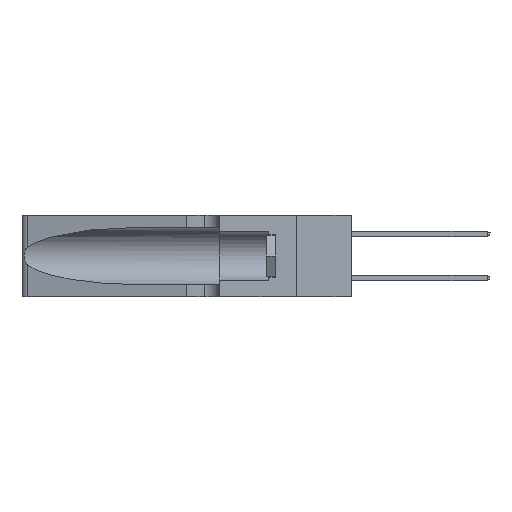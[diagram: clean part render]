
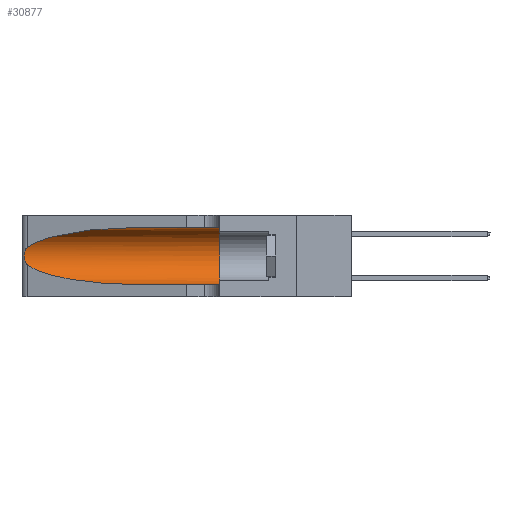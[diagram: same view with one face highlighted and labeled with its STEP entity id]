
A CAD part, left-side view. The second image highlights one B-rep face of the part: STEP entity #30877.
In plain terms, the highlighted cylindrical face has radius 3.308 mm (diameter 6.617 mm), a partial arc.
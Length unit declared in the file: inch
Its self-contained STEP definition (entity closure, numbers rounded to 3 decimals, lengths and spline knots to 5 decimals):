
#311 = CARTESIAN_POINT ( 'NONE',  ( 0.18966, 0.96281, 0.31525 ) ) ;
#879 = ORIENTED_EDGE ( 'NONE', *, *, #33293, .T. ) ;
#2165 = ORIENTED_EDGE ( 'NONE', *, *, #10543, .F. ) ;
#2223 = EDGE_CURVE ( 'NONE', #2775, #30299, #10175, .T. ) ;
#2388 = EDGE_CURVE ( 'NONE', #2775, #19255, #10539, .T. ) ;
#2775 = VERTEX_POINT ( 'NONE', #29743 ) ;
#3473 = EDGE_LOOP ( 'NONE', ( #18449, #19280, #879, #35013, #2165, #21034 ) ) ;
#5345 = CARTESIAN_POINT ( 'NONE',  ( 0.25787, 1.23484, 0.2124 ) ) ;
#5373 = DIRECTION ( 'NONE',  ( 0., -1., 0. ) ) ;
#5460 = DIRECTION ( 'NONE',  ( 0., -1., 0. ) ) ;
#7367 = CARTESIAN_POINT ( 'NONE',  ( 0.1305, 0.72297, 0.05475 ) ) ;
#8260 = CARTESIAN_POINT ( 'NONE',  ( 0.26018, 1.23835, 0.19895 ) ) ;
#8306 = CARTESIAN_POINT ( 'NONE',  ( 0.25487, 1.22718, 0.14631 ) ) ;
#9261 = CARTESIAN_POINT ( 'NONE',  ( 0.18966, 0.96281, 0.05475 ) ) ;
#9454 = FACE_OUTER_BOUND ( 'NONE', #3473, .T. ) ;
#10175 = LINE ( 'NONE', #22093, #12773 ) ;
#10539 =( BOUNDED_CURVE ( )  B_SPLINE_CURVE ( 3, ( #28117, #311, #17195, #30842 ),
 .UNSPECIFIED., .F., .F. ) 
 B_SPLINE_CURVE_WITH_KNOTS ( ( 4, 4 ),
 ( 1.5708, 2.84003 ),
 .UNSPECIFIED. ) 
 CURVE ( )  GEOMETRIC_REPRESENTATION_ITEM ( )  RATIONAL_B_SPLINE_CURVE ( ( 1., 0.87, 0.87, 1. ) ) 
 REPRESENTATION_ITEM ( '' )  );
#10543 = EDGE_CURVE ( 'NONE', #30299, #10990, #32500, .T. ) ;
#10990 = VERTEX_POINT ( 'NONE', #35467 ) ;
#11045 = CARTESIAN_POINT ( 'NONE',  ( 0.26075, 1.23896, 0.178 ) ) ;
#11640 =( BOUNDED_CURVE ( )  B_SPLINE_CURVE ( 3, ( #17498, #33737, #9261, #28424 ),
 .UNSPECIFIED., .F., .T. ) 
 B_SPLINE_CURVE_WITH_KNOTS ( ( 4, 4 ),
 ( 3.44316, 4.71239 ),
 .UNSPECIFIED. ) 
 CURVE ( )  GEOMETRIC_REPRESENTATION_ITEM ( )  RATIONAL_B_SPLINE_CURVE ( ( 1., 0.87, 0.87, 1. ) ) 
 REPRESENTATION_ITEM ( '' )  );
#11899 = AXIS2_PLACEMENT_3D ( 'NONE', #30862, #14536, #33576 ) ;
#12773 = VECTOR ( 'NONE', #5460, 39.37008 ) ;
#13812 = CARTESIAN_POINT ( 'NONE',  ( 0.25856, 1.23593, 0.16098 ) ) ;
#14536 = DIRECTION ( 'NONE',  ( 0., 1., 0. ) ) ;
#15426 = EDGE_CURVE ( 'NONE', #20231, #10990, #32007, .T. ) ;
#15476 = DIRECTION ( 'NONE',  ( 0., 0., -1. ) ) ;
#16509 = CARTESIAN_POINT ( 'NONE',  ( 0.25555, 1.22994, 0.2215 ) ) ;
#16623 = CARTESIAN_POINT ( 'NONE',  ( 0.25639, 1.23186, 0.15144 ) ) ;
#17195 = CARTESIAN_POINT ( 'NONE',  ( 0.2373, 1.15595, 0.28018 ) ) ;
#17498 = CARTESIAN_POINT ( 'NONE',  ( 0.25487, 1.22718, 0.14631 ) ) ;
#17573 = VECTOR ( 'NONE', #22804, 39.37008 ) ;
#18077 = B_SPLINE_CURVE_WITH_KNOTS ( 'NONE', 3,
 ( #19250, #16509, #21989, #5345, #24711, #8260, #27418, #11045, #30160, #13812, #32869, #16623, #35623, #19364 ),
 .UNSPECIFIED., .F., .F.,
 ( 4, 2, 2, 2, 2, 2, 4 ),
 ( 0., 0.00027, 0.00053, 0.00107, 0.0016, 0.00187, 0.00214 ),
 .UNSPECIFIED. ) ;
#18449 = ORIENTED_EDGE ( 'NONE', *, *, #2388, .T. ) ;
#19240 = VERTEX_POINT ( 'NONE', #8306 ) ;
#19250 = CARTESIAN_POINT ( 'NONE',  ( 0.25487, 1.22718, 0.22369 ) ) ;
#19255 = VERTEX_POINT ( 'NONE', #30317 ) ;
#19280 = ORIENTED_EDGE ( 'NONE', *, *, #26374, .T. ) ;
#19364 = CARTESIAN_POINT ( 'NONE',  ( 0.25487, 1.22718, 0.14631 ) ) ;
#20064 = CARTESIAN_POINT ( 'NONE',  ( 0.1305, 1.61858, 0.05475 ) ) ;
#20231 = VERTEX_POINT ( 'NONE', #7367 ) ;
#21034 = ORIENTED_EDGE ( 'NONE', *, *, #2223, .F. ) ;
#21989 = CARTESIAN_POINT ( 'NONE',  ( 0.25639, 1.23184, 0.21858 ) ) ;
#22093 = CARTESIAN_POINT ( 'NONE',  ( 0.1305, 1.61858, 0.31525 ) ) ;
#22804 = DIRECTION ( 'NONE',  ( 0., -1., 0. ) ) ;
#23384 = AXIS2_PLACEMENT_3D ( 'NONE', #24738, #5373, #15476 ) ;
#24711 = CARTESIAN_POINT ( 'NONE',  ( 0.25854, 1.2359, 0.20912 ) ) ;
#24738 = CARTESIAN_POINT ( 'NONE',  ( 0.1305, 1.61858, 0.185 ) ) ;
#26374 = EDGE_CURVE ( 'NONE', #19255, #19240, #18077, .T. ) ;
#27418 = CARTESIAN_POINT ( 'NONE',  ( 0.26075, 1.23896, 0.19203 ) ) ;
#28117 = CARTESIAN_POINT ( 'NONE',  ( 0.1305, 0.72297, 0.31525 ) ) ;
#28424 = CARTESIAN_POINT ( 'NONE',  ( 0.1305, 0.72297, 0.05475 ) ) ;
#29743 = CARTESIAN_POINT ( 'NONE',  ( 0.1305, 0.72297, 0.31525 ) ) ;
#30160 = CARTESIAN_POINT ( 'NONE',  ( 0.26017, 1.23833, 0.17102 ) ) ;
#30299 = VERTEX_POINT ( 'NONE', #33301 ) ;
#30317 = CARTESIAN_POINT ( 'NONE',  ( 0.25487, 1.22718, 0.22369 ) ) ;
#30426 = CYLINDRICAL_SURFACE ( 'NONE', #23384, 0.13025 ) ;
#30842 = CARTESIAN_POINT ( 'NONE',  ( 0.25487, 1.22718, 0.22369 ) ) ;
#30862 = CARTESIAN_POINT ( 'NONE',  ( 0.1305, 0.35, 0.185 ) ) ;
#30877 = ADVANCED_FACE ( 'NONE', ( #9454 ), #30426, .F. ) ;
#32007 = LINE ( 'NONE', #20064, #17573 ) ;
#32500 = CIRCLE ( 'NONE', #11899, 0.13025 ) ;
#32869 = CARTESIAN_POINT ( 'NONE',  ( 0.25789, 1.23486, 0.15765 ) ) ;
#33293 = EDGE_CURVE ( 'NONE', #19240, #20231, #11640, .T. ) ;
#33301 = CARTESIAN_POINT ( 'NONE',  ( 0.1305, 0.35, 0.31525 ) ) ;
#33576 = DIRECTION ( 'NONE',  ( 0., 0., 1. ) ) ;
#33737 = CARTESIAN_POINT ( 'NONE',  ( 0.2373, 1.15595, 0.08982 ) ) ;
#35013 = ORIENTED_EDGE ( 'NONE', *, *, #15426, .T. ) ;
#35467 = CARTESIAN_POINT ( 'NONE',  ( 0.1305, 0.35, 0.05475 ) ) ;
#35623 = CARTESIAN_POINT ( 'NONE',  ( 0.25555, 1.22993, 0.14849 ) ) ;
